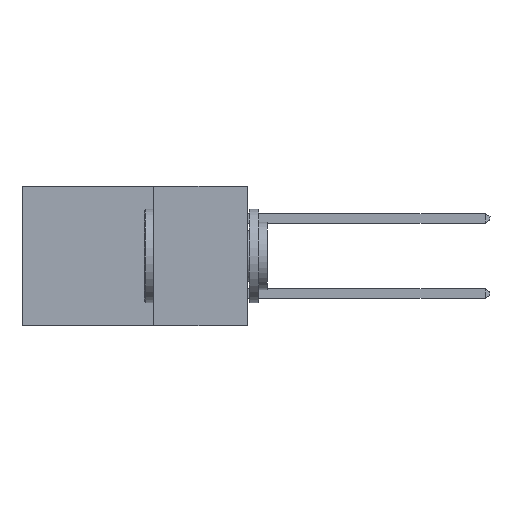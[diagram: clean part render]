
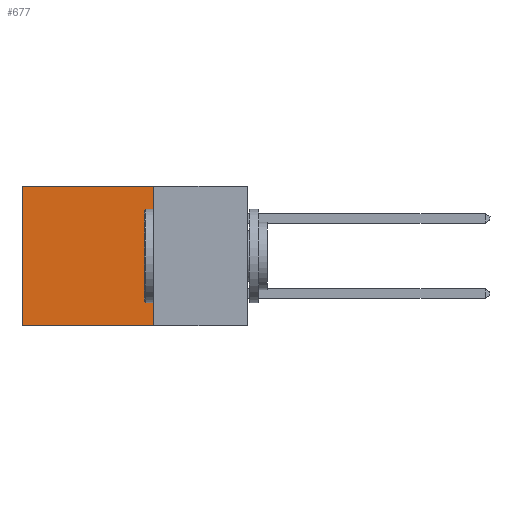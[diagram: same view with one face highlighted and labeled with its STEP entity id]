
A CAD part, left-side view. The second image highlights one B-rep face of the part: STEP entity #677.
In plain terms, the highlighted planar face has unit normal (-1, 0, 0).
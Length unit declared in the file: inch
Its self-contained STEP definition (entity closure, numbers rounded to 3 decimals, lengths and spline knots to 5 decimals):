
#171 = ORIENTED_EDGE ( 'NONE', *, *, #1386, .F. ) ;
#297 = FACE_OUTER_BOUND ( 'NONE', #9415, .T. ) ;
#677 = ADVANCED_FACE ( 'NONE', ( #297 ), #3481, .F. ) ;
#1045 = ORIENTED_EDGE ( 'NONE', *, *, #7121, .T. ) ;
#1173 = DIRECTION ( 'NONE',  ( 0., 0., -1. ) ) ;
#1214 = VECTOR ( 'NONE', #6318, 39.37008 ) ;
#1221 = LINE ( 'NONE', #8303, #5349 ) ;
#1242 = CARTESIAN_POINT ( 'NONE',  ( 0.2615, 0.25, 0. ) ) ;
#1386 = EDGE_CURVE ( 'NONE', #8440, #4947, #1221, .T. ) ;
#1820 = EDGE_CURVE ( 'NONE', #4947, #8298, #9436, .T. ) ;
#2224 = VECTOR ( 'NONE', #4110, 39.37008 ) ;
#2704 = LINE ( 'NONE', #8985, #5603 ) ;
#2856 = DIRECTION ( 'NONE',  ( 0., 1., 0. ) ) ;
#3481 = PLANE ( 'NONE',  #6840 ) ;
#4098 = DIRECTION ( 'NONE',  ( 1., 0., 0. ) ) ;
#4110 = DIRECTION ( 'NONE',  ( 0., 0., -1. ) ) ;
#4947 = VERTEX_POINT ( 'NONE', #9451 ) ;
#5349 = VECTOR ( 'NONE', #1173, 39.37008 ) ;
#5603 = VECTOR ( 'NONE', #2856, 39.37008 ) ;
#5674 = LINE ( 'NONE', #8832, #2224 ) ;
#6318 = DIRECTION ( 'NONE',  ( 0., 1., 0. ) ) ;
#6381 = VERTEX_POINT ( 'NONE', #6992 ) ;
#6648 = CARTESIAN_POINT ( 'NONE',  ( 0.2615, 0.25, -0.37 ) ) ;
#6840 = AXIS2_PLACEMENT_3D ( 'NONE', #6648, #4098, #9657 ) ;
#6992 = CARTESIAN_POINT ( 'NONE',  ( 0.2615, 0.6, 0. ) ) ;
#7121 = EDGE_CURVE ( 'NONE', #6381, #8298, #5674, .T. ) ;
#7874 = CARTESIAN_POINT ( 'NONE',  ( 0.2615, 0.25, -0.37 ) ) ;
#8298 = VERTEX_POINT ( 'NONE', #8943 ) ;
#8303 = CARTESIAN_POINT ( 'NONE',  ( 0.2615, 0.25, -0.37 ) ) ;
#8440 = VERTEX_POINT ( 'NONE', #1242 ) ;
#8443 = ORIENTED_EDGE ( 'NONE', *, *, #8901, .T. ) ;
#8832 = CARTESIAN_POINT ( 'NONE',  ( 0.2615, 0.6, -0.37 ) ) ;
#8901 = EDGE_CURVE ( 'NONE', #8440, #6381, #2704, .T. ) ;
#8943 = CARTESIAN_POINT ( 'NONE',  ( 0.2615, 0.6, -0.37 ) ) ;
#8985 = CARTESIAN_POINT ( 'NONE',  ( 0.2615, 0.25, 0. ) ) ;
#9415 = EDGE_LOOP ( 'NONE', ( #1045, #9772, #171, #8443 ) ) ;
#9436 = LINE ( 'NONE', #7874, #1214 ) ;
#9451 = CARTESIAN_POINT ( 'NONE',  ( 0.2615, 0.25, -0.37 ) ) ;
#9657 = DIRECTION ( 'NONE',  ( 0., 0., -1. ) ) ;
#9772 = ORIENTED_EDGE ( 'NONE', *, *, #1820, .F. ) ;
